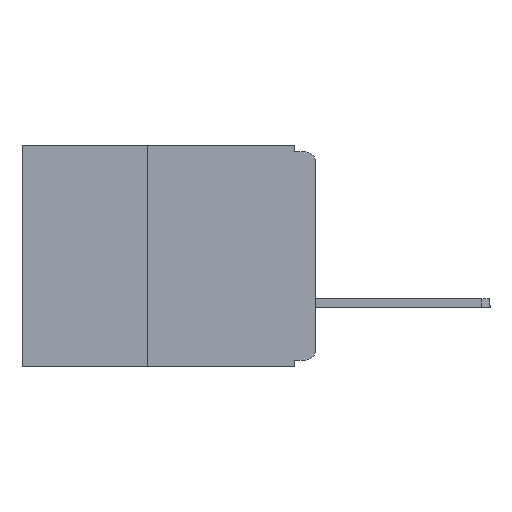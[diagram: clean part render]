
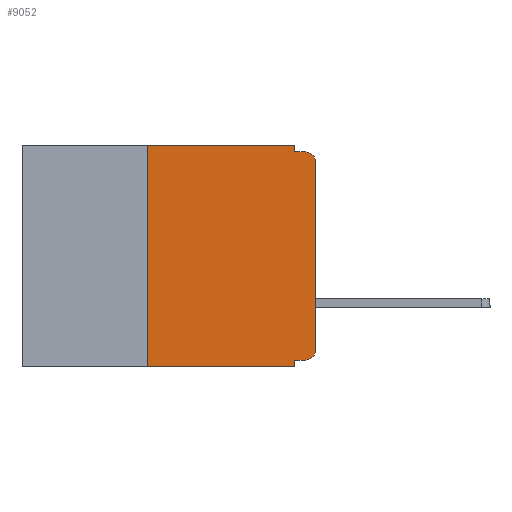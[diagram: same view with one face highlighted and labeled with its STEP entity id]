
A CAD part, left-side view. The second image highlights one B-rep face of the part: STEP entity #9052.
In plain terms, the highlighted planar face has unit normal (-1, 0, 0).
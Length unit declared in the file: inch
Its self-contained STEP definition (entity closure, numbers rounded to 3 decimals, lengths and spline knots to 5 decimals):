
#2 = EDGE_CURVE ( 'NONE', #1739, #467, #6961, .T. ) ;
#98 = VERTEX_POINT ( 'NONE', #11899 ) ;
#443 = CARTESIAN_POINT ( 'NONE',  ( 0., 0.031, -0.33 ) ) ;
#467 = VERTEX_POINT ( 'NONE', #3486 ) ;
#1137 = EDGE_CURVE ( 'NONE', #7048, #4152, #2585, .T. ) ;
#1176 = PLANE ( 'NONE',  #3092 ) ;
#1221 = EDGE_CURVE ( 'NONE', #15306, #4360, #11767, .T. ) ;
#1334 = ORIENTED_EDGE ( 'NONE', *, *, #12534, .F. ) ;
#1429 = LINE ( 'NONE', #9812, #8358 ) ;
#1541 = ORIENTED_EDGE ( 'NONE', *, *, #4890, .T. ) ;
#1559 = CARTESIAN_POINT ( 'NONE',  ( 0., 0.25, -0.33 ) ) ;
#1706 = EDGE_CURVE ( 'NONE', #7048, #5264, #17097, .T. ) ;
#1739 = VERTEX_POINT ( 'NONE', #8323 ) ;
#2113 = LINE ( 'NONE', #11754, #9458 ) ;
#2217 = VERTEX_POINT ( 'NONE', #10616 ) ;
#2296 = DIRECTION ( 'NONE',  ( 0., -1., 0. ) ) ;
#2585 = CIRCLE ( 'NONE', #3813, 0.015 ) ;
#3032 = AXIS2_PLACEMENT_3D ( 'NONE', #8678, #8622, #8561 ) ;
#3092 = AXIS2_PLACEMENT_3D ( 'NONE', #10825, #12120, #3993 ) ;
#3281 = VECTOR ( 'NONE', #2296, 39.37008 ) ;
#3486 = CARTESIAN_POINT ( 'NONE',  ( 0., 0.031, 0. ) ) ;
#3534 = ORIENTED_EDGE ( 'NONE', *, *, #1221, .T. ) ;
#3547 = VECTOR ( 'NONE', #4016, 39.37008 ) ;
#3549 = FACE_OUTER_BOUND ( 'NONE', #13141, .T. ) ;
#3600 = DIRECTION ( 'NONE',  ( 0., 0., 1. ) ) ;
#3750 = ORIENTED_EDGE ( 'NONE', *, *, #2, .F. ) ;
#3813 = AXIS2_PLACEMENT_3D ( 'NONE', #16243, #16242, #16224 ) ;
#3993 = DIRECTION ( 'NONE',  ( 0., 0., -1. ) ) ;
#4016 = DIRECTION ( 'NONE',  ( 0., 0., -1. ) ) ;
#4152 = VERTEX_POINT ( 'NONE', #8279 ) ;
#4360 = VERTEX_POINT ( 'NONE', #443 ) ;
#4804 = CARTESIAN_POINT ( 'NONE',  ( 0., 0.031, -0.01 ) ) ;
#4890 = EDGE_CURVE ( 'NONE', #98, #2217, #15684, .T. ) ;
#5250 = DIRECTION ( 'NONE',  ( 0., 1., 0. ) ) ;
#5264 = VERTEX_POINT ( 'NONE', #14808 ) ;
#5716 = ORIENTED_EDGE ( 'NONE', *, *, #15566, .T. ) ;
#5882 = EDGE_CURVE ( 'NONE', #15306, #1739, #1429, .T. ) ;
#6459 = CARTESIAN_POINT ( 'NONE',  ( 0., 0., -0.01 ) ) ;
#6737 = CARTESIAN_POINT ( 'NONE',  ( 0., 0.031, 0. ) ) ;
#6925 = CARTESIAN_POINT ( 'NONE',  ( 0., 0.437, 0. ) ) ;
#6961 = LINE ( 'NONE', #6925, #3281 ) ;
#7048 = VERTEX_POINT ( 'NONE', #15969 ) ;
#7640 = LINE ( 'NONE', #6737, #3547 ) ;
#7882 = DIRECTION ( 'NONE',  ( 0., -1., 0. ) ) ;
#8279 = CARTESIAN_POINT ( 'NONE',  ( 0., 0., -0.305 ) ) ;
#8323 = CARTESIAN_POINT ( 'NONE',  ( 0., 0.25, 0. ) ) ;
#8358 = VECTOR ( 'NONE', #9728, 39.37008 ) ;
#8561 = DIRECTION ( 'NONE',  ( 0., 0., -1. ) ) ;
#8622 = DIRECTION ( 'NONE',  ( -1., 0., 0. ) ) ;
#8641 = LINE ( 'NONE', #6459, #15309 ) ;
#8678 = CARTESIAN_POINT ( 'NONE',  ( 0., 0.015, -0.025 ) ) ;
#8881 = VECTOR ( 'NONE', #10221, 39.37008 ) ;
#9052 = ADVANCED_FACE ( 'NONE', ( #3549 ), #1176, .F. ) ;
#9305 = CARTESIAN_POINT ( 'NONE',  ( 0., 0., -0.32 ) ) ;
#9458 = VECTOR ( 'NONE', #3600, 39.37008 ) ;
#9728 = DIRECTION ( 'NONE',  ( 0., 0., 1. ) ) ;
#9812 = CARTESIAN_POINT ( 'NONE',  ( 0., 0.25, -0.33 ) ) ;
#10221 = DIRECTION ( 'NONE',  ( 0., 0., -1. ) ) ;
#10384 = ORIENTED_EDGE ( 'NONE', *, *, #12212, .F. ) ;
#10616 = CARTESIAN_POINT ( 'NONE',  ( 0., 0.015, -0.01 ) ) ;
#10639 = ORIENTED_EDGE ( 'NONE', *, *, #1137, .T. ) ;
#10776 = VERTEX_POINT ( 'NONE', #4804 ) ;
#10825 = CARTESIAN_POINT ( 'NONE',  ( 0., 0.437, 0. ) ) ;
#11367 = VECTOR ( 'NONE', #12049, 39.37008 ) ;
#11754 = CARTESIAN_POINT ( 'NONE',  ( 0., 0., 0. ) ) ;
#11767 = LINE ( 'NONE', #15805, #11367 ) ;
#11899 = CARTESIAN_POINT ( 'NONE',  ( 0., 0., -0.025 ) ) ;
#12049 = DIRECTION ( 'NONE',  ( 0., -1., 0. ) ) ;
#12120 = DIRECTION ( 'NONE',  ( 1., 0., 0. ) ) ;
#12212 = EDGE_CURVE ( 'NONE', #467, #10776, #7640, .T. ) ;
#12534 = EDGE_CURVE ( 'NONE', #5264, #4360, #12849, .T. ) ;
#12849 = LINE ( 'NONE', #15465, #8881 ) ;
#13141 = EDGE_LOOP ( 'NONE', ( #5716, #1541, #15551, #10384, #3750, #16804, #3534, #1334, #15341, #10639 ) ) ;
#13218 = EDGE_CURVE ( 'NONE', #10776, #2217, #8641, .T. ) ;
#13578 = VECTOR ( 'NONE', #5250, 39.37008 ) ;
#14808 = CARTESIAN_POINT ( 'NONE',  ( 0., 0.031, -0.32 ) ) ;
#15306 = VERTEX_POINT ( 'NONE', #1559 ) ;
#15309 = VECTOR ( 'NONE', #7882, 39.37008 ) ;
#15341 = ORIENTED_EDGE ( 'NONE', *, *, #1706, .F. ) ;
#15465 = CARTESIAN_POINT ( 'NONE',  ( 0., 0.031, -0.33 ) ) ;
#15551 = ORIENTED_EDGE ( 'NONE', *, *, #13218, .F. ) ;
#15566 = EDGE_CURVE ( 'NONE', #4152, #98, #2113, .T. ) ;
#15684 = CIRCLE ( 'NONE', #3032, 0.015 ) ;
#15805 = CARTESIAN_POINT ( 'NONE',  ( 0., 0.437, -0.33 ) ) ;
#15969 = CARTESIAN_POINT ( 'NONE',  ( 0., 0.015, -0.32 ) ) ;
#16224 = DIRECTION ( 'NONE',  ( 0., 0., -1. ) ) ;
#16242 = DIRECTION ( 'NONE',  ( -1., 0., 0. ) ) ;
#16243 = CARTESIAN_POINT ( 'NONE',  ( 0., 0.015, -0.305 ) ) ;
#16804 = ORIENTED_EDGE ( 'NONE', *, *, #5882, .F. ) ;
#17097 = LINE ( 'NONE', #9305, #13578 ) ;
